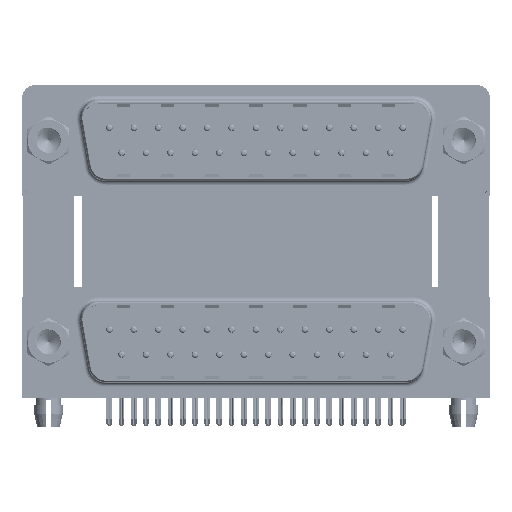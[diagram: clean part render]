
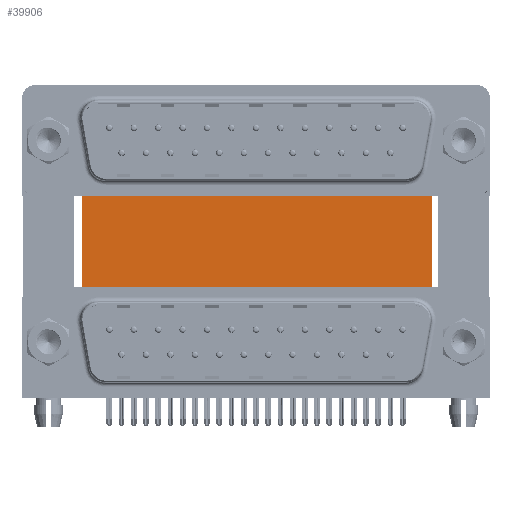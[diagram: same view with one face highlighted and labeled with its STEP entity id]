
A CAD part, top view. The second image highlights one B-rep face of the part: STEP entity #39906.
In plain terms, the highlighted planar face has unit normal (0, 0, 1).
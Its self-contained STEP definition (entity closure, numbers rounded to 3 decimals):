
#126 = VECTOR ( 'NONE', #9850, 1000. ) ;
#707 = VECTOR ( 'NONE', #29125, 1000. ) ;
#768 = EDGE_CURVE ( 'NONE', #23194, #29846, #26894, .T. ) ;
#930 = DIRECTION ( 'NONE',  ( -1., 0., 0. ) ) ;
#2089 = VECTOR ( 'NONE', #23284, 1000. ) ;
#5045 = AXIS2_PLACEMENT_3D ( 'NONE', #44131, #40584, #930 ) ;
#5860 = EDGE_CURVE ( 'NONE', #46858, #29846, #46892, .T. ) ;
#9850 = DIRECTION ( 'NONE',  ( 1., 0., 0. ) ) ;
#10794 = EDGE_CURVE ( 'NONE', #40035, #46858, #34192, .T. ) ;
#12385 = DIRECTION ( 'NONE',  ( 0., -1., 0. ) ) ;
#13204 = CARTESIAN_POINT ( 'NONE',  ( 3.79, 16.585, -12. ) ) ;
#13254 = CARTESIAN_POINT ( 'NONE',  ( 3.79, 16.585, -12. ) ) ;
#14707 = EDGE_LOOP ( 'NONE', ( #18845, #27051, #46658, #25876 ) ) ;
#18334 = CARTESIAN_POINT ( 'NONE',  ( 3.79, -3.735, -12. ) ) ;
#18845 = ORIENTED_EDGE ( 'NONE', *, *, #5860, .T. ) ;
#23194 = VERTEX_POINT ( 'NONE', #45015 ) ;
#23284 = DIRECTION ( 'NONE',  ( 0., -1., 0. ) ) ;
#23422 = EDGE_CURVE ( 'NONE', #40035, #23194, #24141, .T. ) ;
#24141 = LINE ( 'NONE', #13204, #126 ) ;
#25876 = ORIENTED_EDGE ( 'NONE', *, *, #10794, .T. ) ;
#26894 = LINE ( 'NONE', #33302, #27802 ) ;
#27051 = ORIENTED_EDGE ( 'NONE', *, *, #768, .F. ) ;
#27802 = VECTOR ( 'NONE', #12385, 1000. ) ;
#29125 = DIRECTION ( 'NONE',  ( 1., 0., 0. ) ) ;
#29846 = VERTEX_POINT ( 'NONE', #42820 ) ;
#33302 = CARTESIAN_POINT ( 'NONE',  ( 43.43, 16.585, -12. ) ) ;
#33940 = FACE_OUTER_BOUND ( 'NONE', #14707, .T. ) ;
#34192 = LINE ( 'NONE', #38229, #2089 ) ;
#37729 = PLANE ( 'NONE',  #5045 ) ;
#38229 = CARTESIAN_POINT ( 'NONE',  ( 3.79, 16.585, -12. ) ) ;
#39906 = ADVANCED_FACE ( 'NONE', ( #33940 ), #37729, .F. ) ;
#40021 = CARTESIAN_POINT ( 'NONE',  ( 3.79, -3.735, -12. ) ) ;
#40035 = VERTEX_POINT ( 'NONE', #13254 ) ;
#40584 = DIRECTION ( 'NONE',  ( 0., 0., -1. ) ) ;
#42820 = CARTESIAN_POINT ( 'NONE',  ( 43.43, -3.735, -12. ) ) ;
#44131 = CARTESIAN_POINT ( 'NONE',  ( 3.79, 16.585, -12. ) ) ;
#45015 = CARTESIAN_POINT ( 'NONE',  ( 43.43, 16.585, -12. ) ) ;
#46658 = ORIENTED_EDGE ( 'NONE', *, *, #23422, .F. ) ;
#46858 = VERTEX_POINT ( 'NONE', #18334 ) ;
#46892 = LINE ( 'NONE', #40021, #707 ) ;
